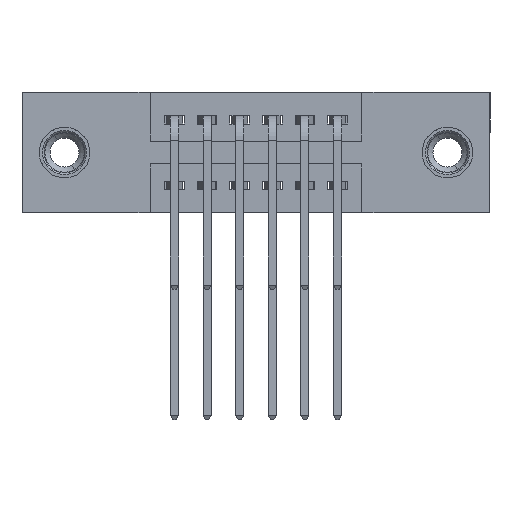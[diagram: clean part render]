
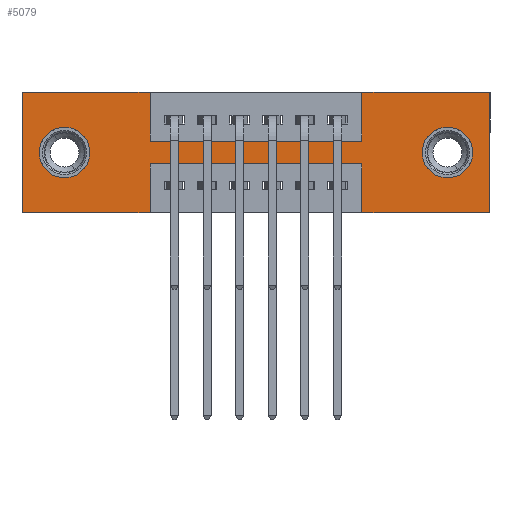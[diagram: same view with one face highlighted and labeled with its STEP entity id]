
A CAD part, front view. The second image highlights one B-rep face of the part: STEP entity #5079.
In plain terms, the highlighted planar face has unit normal (0, -1, 0).
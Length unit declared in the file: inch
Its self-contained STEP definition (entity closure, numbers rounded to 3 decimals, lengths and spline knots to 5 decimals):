
#307 = VECTOR ( 'NONE', #10417, 39.37008 ) ;
#357 = VERTEX_POINT ( 'NONE', #12663 ) ;
#460 = CARTESIAN_POINT ( 'NONE',  ( 0., 0., 0. ) ) ;
#618 = DIRECTION ( 'NONE',  ( 0., 0., -1. ) ) ;
#625 = CARTESIAN_POINT ( 'NONE',  ( 0., 0., -0.37 ) ) ;
#646 = CIRCLE ( 'NONE', #7721, 0.078 ) ;
#647 = CIRCLE ( 'NONE', #4291, 0.078 ) ;
#801 = EDGE_LOOP ( 'NONE', ( #2126, #4710 ) ) ;
#818 = LINE ( 'NONE', #8605, #6082 ) ;
#954 = VERTEX_POINT ( 'NONE', #13020 ) ;
#1061 = LINE ( 'NONE', #460, #6340 ) ;
#1063 = EDGE_CURVE ( 'NONE', #2007, #4875, #646, .T. ) ;
#1109 = CARTESIAN_POINT ( 'NONE',  ( 0., 0., -0.37 ) ) ;
#1129 = ORIENTED_EDGE ( 'NONE', *, *, #11967, .F. ) ;
#1452 = CARTESIAN_POINT ( 'NONE',  ( 1.0425, 0., 0. ) ) ;
#1510 = ORIENTED_EDGE ( 'NONE', *, *, #8387, .F. ) ;
#1649 = DIRECTION ( 'NONE',  ( 0., 0., -1. ) ) ;
#1749 = LINE ( 'NONE', #6519, #10033 ) ;
#1751 = EDGE_CURVE ( 'NONE', #8564, #954, #818, .T. ) ;
#1761 = CARTESIAN_POINT ( 'NONE',  ( 0., 0., 0. ) ) ;
#1917 = EDGE_CURVE ( 'NONE', #12074, #4683, #4429, .T. ) ;
#1986 = EDGE_CURVE ( 'NONE', #4875, #2007, #647, .T. ) ;
#2000 = EDGE_CURVE ( 'NONE', #4073, #5865, #11390, .T. ) ;
#2007 = VERTEX_POINT ( 'NONE', #5225 ) ;
#2045 = CARTESIAN_POINT ( 'NONE',  ( 0.3925, 0., -0.37 ) ) ;
#2126 = ORIENTED_EDGE ( 'NONE', *, *, #1986, .T. ) ;
#2204 = LINE ( 'NONE', #7841, #12865 ) ;
#2297 = AXIS2_PLACEMENT_3D ( 'NONE', #625, #9990, #3791 ) ;
#2402 = LINE ( 'NONE', #8837, #7687 ) ;
#2640 = DIRECTION ( 'NONE',  ( 0., 1., 0. ) ) ;
#2707 = CARTESIAN_POINT ( 'NONE',  ( 0.13, 0., -0.185 ) ) ;
#2725 = PLANE ( 'NONE',  #2297 ) ;
#2758 = CARTESIAN_POINT ( 'NONE',  ( 1.0425, 0., -0.15 ) ) ;
#2984 = VERTEX_POINT ( 'NONE', #6946 ) ;
#3094 = LINE ( 'NONE', #2045, #8339 ) ;
#3534 = ORIENTED_EDGE ( 'NONE', *, *, #7712, .T. ) ;
#3661 = DIRECTION ( 'NONE',  ( 0., 0., 1. ) ) ;
#3763 = ORIENTED_EDGE ( 'NONE', *, *, #4999, .F. ) ;
#3782 = VERTEX_POINT ( 'NONE', #9422 ) ;
#3791 = DIRECTION ( 'NONE',  ( 0., 0., -1. ) ) ;
#3945 = EDGE_CURVE ( 'NONE', #5763, #8564, #1749, .T. ) ;
#4073 = VERTEX_POINT ( 'NONE', #6717 ) ;
#4111 = VECTOR ( 'NONE', #11625, 39.37008 ) ;
#4172 = ORIENTED_EDGE ( 'NONE', *, *, #9815, .F. ) ;
#4291 = AXIS2_PLACEMENT_3D ( 'NONE', #7882, #12166, #12158 ) ;
#4343 = FACE_BOUND ( 'NONE', #801, .T. ) ;
#4429 = LINE ( 'NONE', #1452, #4111 ) ;
#4631 = EDGE_CURVE ( 'NONE', #954, #12074, #6861, .T. ) ;
#4683 = VERTEX_POINT ( 'NONE', #13394 ) ;
#4710 = ORIENTED_EDGE ( 'NONE', *, *, #1063, .T. ) ;
#4732 = DIRECTION ( 'NONE',  ( 0., 1., 0. ) ) ;
#4759 = CARTESIAN_POINT ( 'NONE',  ( 1.435, 0., 0. ) ) ;
#4875 = VERTEX_POINT ( 'NONE', #11732 ) ;
#4987 = ORIENTED_EDGE ( 'NONE', *, *, #8942, .F. ) ;
#4992 = CIRCLE ( 'NONE', #10216, 0.078 ) ;
#4999 = EDGE_CURVE ( 'NONE', #13118, #5763, #2204, .T. ) ;
#5020 = EDGE_CURVE ( 'NONE', #11973, #3782, #4992, .T. ) ;
#5059 = CARTESIAN_POINT ( 'NONE',  ( 1.0425, 0., -0.22 ) ) ;
#5061 = ORIENTED_EDGE ( 'NONE', *, *, #1751, .F. ) ;
#5079 = ADVANCED_FACE ( 'NONE', ( #7168, #4343, #12428 ), #2725, .T. ) ;
#5184 = DIRECTION ( 'NONE',  ( 1., 0., 0. ) ) ;
#5225 = CARTESIAN_POINT ( 'NONE',  ( 0.13, 0., -0.263 ) ) ;
#5339 = ORIENTED_EDGE ( 'NONE', *, *, #3945, .F. ) ;
#5615 = EDGE_CURVE ( 'NONE', #4683, #11174, #1061, .T. ) ;
#5760 = CARTESIAN_POINT ( 'NONE',  ( 1.305, 0., -0.263 ) ) ;
#5763 = VERTEX_POINT ( 'NONE', #1761 ) ;
#5865 = VERTEX_POINT ( 'NONE', #5059 ) ;
#6082 = VECTOR ( 'NONE', #7997, 39.37008 ) ;
#6275 = ORIENTED_EDGE ( 'NONE', *, *, #4631, .F. ) ;
#6332 = CARTESIAN_POINT ( 'NONE',  ( 0.3925, 0., -0.37 ) ) ;
#6340 = VECTOR ( 'NONE', #6813, 39.37008 ) ;
#6519 = CARTESIAN_POINT ( 'NONE',  ( 0., 0., 0. ) ) ;
#6624 = VECTOR ( 'NONE', #13148, 39.37008 ) ;
#6717 = CARTESIAN_POINT ( 'NONE',  ( 1.0425, 0., -0.37 ) ) ;
#6730 = ORIENTED_EDGE ( 'NONE', *, *, #9871, .F. ) ;
#6813 = DIRECTION ( 'NONE',  ( 1., 0., 0. ) ) ;
#6861 = LINE ( 'NONE', #10336, #11955 ) ;
#6923 = DIRECTION ( 'NONE',  ( 1., 0., 0. ) ) ;
#6946 = CARTESIAN_POINT ( 'NONE',  ( 1.435, 0., -0.37 ) ) ;
#6950 = DIRECTION ( 'NONE',  ( 0., 1., 0. ) ) ;
#7071 = EDGE_LOOP ( 'NONE', ( #3534, #13124 ) ) ;
#7168 = FACE_BOUND ( 'NONE', #7071, .T. ) ;
#7274 = AXIS2_PLACEMENT_3D ( 'NONE', #12996, #6950, #618 ) ;
#7278 = VERTEX_POINT ( 'NONE', #6332 ) ;
#7348 = DIRECTION ( 'NONE',  ( 0., 0., -1. ) ) ;
#7687 = VECTOR ( 'NONE', #9847, 39.37008 ) ;
#7712 = EDGE_CURVE ( 'NONE', #3782, #11973, #12203, .T. ) ;
#7719 = VECTOR ( 'NONE', #9402, 39.37008 ) ;
#7721 = AXIS2_PLACEMENT_3D ( 'NONE', #2707, #4732, #7898 ) ;
#7841 = CARTESIAN_POINT ( 'NONE',  ( 0., 0., 0. ) ) ;
#7882 = CARTESIAN_POINT ( 'NONE',  ( 0.13, 0., -0.185 ) ) ;
#7898 = DIRECTION ( 'NONE',  ( 0., 0., 1. ) ) ;
#7997 = DIRECTION ( 'NONE',  ( 0., 0., -1. ) ) ;
#8339 = VECTOR ( 'NONE', #7348, 39.37008 ) ;
#8387 = EDGE_CURVE ( 'NONE', #5865, #357, #9311, .T. ) ;
#8517 = CARTESIAN_POINT ( 'NONE',  ( 1.0425, 0., -0.37 ) ) ;
#8564 = VERTEX_POINT ( 'NONE', #10393 ) ;
#8605 = CARTESIAN_POINT ( 'NONE',  ( 0.3925, 0., 0. ) ) ;
#8837 = CARTESIAN_POINT ( 'NONE',  ( 0., 0., -0.37 ) ) ;
#8897 = CARTESIAN_POINT ( 'NONE',  ( 1.305, 0., -0.185 ) ) ;
#8942 = EDGE_CURVE ( 'NONE', #11174, #2984, #12088, .T. ) ;
#9089 = CARTESIAN_POINT ( 'NONE',  ( 0.3925, 0., -0.22 ) ) ;
#9311 = LINE ( 'NONE', #9089, #6624 ) ;
#9402 = DIRECTION ( 'NONE',  ( -1., 0., 0. ) ) ;
#9422 = CARTESIAN_POINT ( 'NONE',  ( 1.305, 0., -0.107 ) ) ;
#9720 = ORIENTED_EDGE ( 'NONE', *, *, #5615, .F. ) ;
#9751 = ORIENTED_EDGE ( 'NONE', *, *, #2000, .F. ) ;
#9815 = EDGE_CURVE ( 'NONE', #357, #7278, #3094, .T. ) ;
#9847 = DIRECTION ( 'NONE',  ( -1., 0., 0. ) ) ;
#9871 = EDGE_CURVE ( 'NONE', #2984, #4073, #10409, .T. ) ;
#9905 = DIRECTION ( 'NONE',  ( 0., 0., -1. ) ) ;
#9974 = ORIENTED_EDGE ( 'NONE', *, *, #1917, .F. ) ;
#9990 = DIRECTION ( 'NONE',  ( 0., -1., 0. ) ) ;
#10033 = VECTOR ( 'NONE', #6923, 39.37008 ) ;
#10216 = AXIS2_PLACEMENT_3D ( 'NONE', #8897, #2640, #9905 ) ;
#10336 = CARTESIAN_POINT ( 'NONE',  ( 0.3925, 0., -0.15 ) ) ;
#10393 = CARTESIAN_POINT ( 'NONE',  ( 0.3925, 0., 0. ) ) ;
#10409 = LINE ( 'NONE', #1109, #7719 ) ;
#10417 = DIRECTION ( 'NONE',  ( 0., 0., 1. ) ) ;
#10643 = CARTESIAN_POINT ( 'NONE',  ( 1.435, 0., 0. ) ) ;
#10749 = VECTOR ( 'NONE', #1649, 39.37008 ) ;
#11174 = VERTEX_POINT ( 'NONE', #10643 ) ;
#11314 = EDGE_LOOP ( 'NONE', ( #4172, #1510, #9751, #6730, #4987, #9720, #9974, #6275, #5061, #5339, #3763, #1129 ) ) ;
#11390 = LINE ( 'NONE', #8517, #307 ) ;
#11605 = CARTESIAN_POINT ( 'NONE',  ( 0., 0., -0.37 ) ) ;
#11625 = DIRECTION ( 'NONE',  ( 0., 0., 1. ) ) ;
#11732 = CARTESIAN_POINT ( 'NONE',  ( 0.13, 0., -0.107 ) ) ;
#11955 = VECTOR ( 'NONE', #5184, 39.37008 ) ;
#11967 = EDGE_CURVE ( 'NONE', #7278, #13118, #2402, .T. ) ;
#11973 = VERTEX_POINT ( 'NONE', #5760 ) ;
#12074 = VERTEX_POINT ( 'NONE', #2758 ) ;
#12088 = LINE ( 'NONE', #4759, #10749 ) ;
#12158 = DIRECTION ( 'NONE',  ( 0., 0., 1. ) ) ;
#12166 = DIRECTION ( 'NONE',  ( 0., 1., 0. ) ) ;
#12203 = CIRCLE ( 'NONE', #7274, 0.078 ) ;
#12428 = FACE_OUTER_BOUND ( 'NONE', #11314, .T. ) ;
#12663 = CARTESIAN_POINT ( 'NONE',  ( 0.3925, 0., -0.22 ) ) ;
#12865 = VECTOR ( 'NONE', #3661, 39.37008 ) ;
#12996 = CARTESIAN_POINT ( 'NONE',  ( 1.305, 0., -0.185 ) ) ;
#13020 = CARTESIAN_POINT ( 'NONE',  ( 0.3925, 0., -0.15 ) ) ;
#13118 = VERTEX_POINT ( 'NONE', #11605 ) ;
#13124 = ORIENTED_EDGE ( 'NONE', *, *, #5020, .T. ) ;
#13148 = DIRECTION ( 'NONE',  ( -1., 0., 0. ) ) ;
#13394 = CARTESIAN_POINT ( 'NONE',  ( 1.0425, 0., 0. ) ) ;
